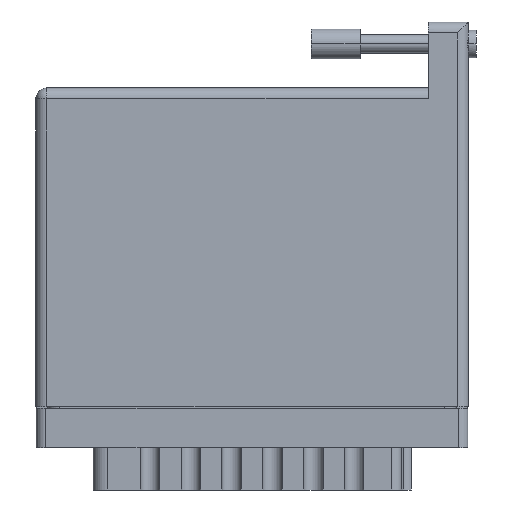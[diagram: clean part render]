
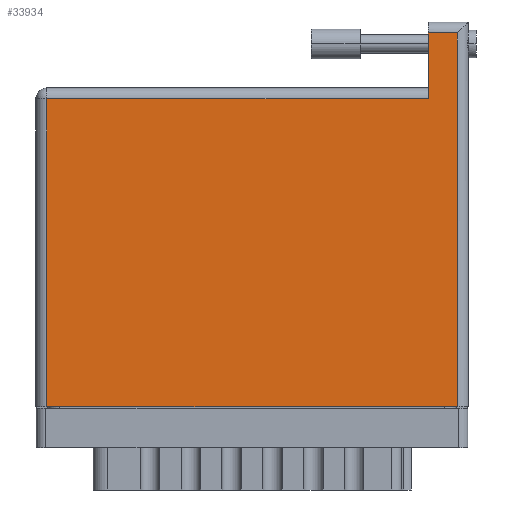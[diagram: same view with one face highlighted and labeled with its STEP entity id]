
A CAD part, front view. The second image highlights one B-rep face of the part: STEP entity #33934.
In plain terms, the highlighted face is planar.
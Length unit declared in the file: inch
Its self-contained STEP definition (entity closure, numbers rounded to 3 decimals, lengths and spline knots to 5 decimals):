
#3398 = CARTESIAN_POINT ( 'NONE',  ( 0., 2.38, 0. ) ) ;
#4438 = ORIENTED_EDGE ( 'NONE', *, *, #32680, .T. ) ;
#5184 = AXIS2_PLACEMENT_3D ( 'NONE', #55172, #81956, #68288 ) ;
#7127 = EDGE_CURVE ( 'NONE', #17863, #19327, #41618, .T. ) ;
#8335 = PLANE ( 'NONE',  #5184 ) ;
#9210 = VERTEX_POINT ( 'NONE', #64380 ) ;
#9655 = ORIENTED_EDGE ( 'NONE', *, *, #7127, .T. ) ;
#12893 = DIRECTION ( 'NONE',  ( 0., -1., 0. ) ) ;
#14380 = ORIENTED_EDGE ( 'NONE', *, *, #60143, .T. ) ;
#15387 = EDGE_LOOP ( 'NONE', ( #14380, #84192, #4438, #9655, #59409, #62923 ) ) ;
#15665 = CARTESIAN_POINT ( 'NONE',  ( 2.685, 0., 0. ) ) ;
#17863 = VERTEX_POINT ( 'NONE', #59185 ) ;
#19327 = VERTEX_POINT ( 'NONE', #15665 ) ;
#20785 = VECTOR ( 'NONE', #63947, 39.37008 ) ;
#22750 = CARTESIAN_POINT ( 'NONE',  ( 2.685, 2.38, 0. ) ) ;
#22816 = VECTOR ( 'NONE', #77597, 39.37008 ) ;
#23633 = CARTESIAN_POINT ( 'NONE',  ( 2.499, 1.96, 0. ) ) ;
#29413 = LINE ( 'NONE', #57463, #50228 ) ;
#31864 = CARTESIAN_POINT ( 'NONE',  ( 0., 0., 0. ) ) ;
#32680 = EDGE_CURVE ( 'NONE', #81911, #17863, #42531, .T. ) ;
#33247 = EDGE_CURVE ( 'NONE', #19327, #50905, #82071, .T. ) ;
#33934 = ADVANCED_FACE ( 'NONE', ( #63229 ), #8335, .F. ) ;
#36500 = DIRECTION ( 'NONE',  ( 0., -1., 0. ) ) ;
#39811 = DIRECTION ( 'NONE',  ( 0., 1., 0. ) ) ;
#41059 = VERTEX_POINT ( 'NONE', #23633 ) ;
#41294 = LINE ( 'NONE', #53736, #79901 ) ;
#41618 = LINE ( 'NONE', #31864, #22816 ) ;
#42531 = LINE ( 'NONE', #79247, #77936 ) ;
#46862 = LINE ( 'NONE', #3398, #20785 ) ;
#50228 = VECTOR ( 'NONE', #36500, 39.37008 ) ;
#50905 = VERTEX_POINT ( 'NONE', #22750 ) ;
#53736 = CARTESIAN_POINT ( 'NONE',  ( 0., 1.96, 0. ) ) ;
#54991 = EDGE_CURVE ( 'NONE', #50905, #9210, #46862, .T. ) ;
#55172 = CARTESIAN_POINT ( 'NONE',  ( 0., 2.03, 0. ) ) ;
#57463 = CARTESIAN_POINT ( 'NONE',  ( 2.499, 2.45, 0. ) ) ;
#59185 = CARTESIAN_POINT ( 'NONE',  ( 0.07, 0., 0. ) ) ;
#59409 = ORIENTED_EDGE ( 'NONE', *, *, #33247, .T. ) ;
#60143 = EDGE_CURVE ( 'NONE', #9210, #41059, #29413, .T. ) ;
#62923 = ORIENTED_EDGE ( 'NONE', *, *, #54991, .T. ) ;
#63229 = FACE_OUTER_BOUND ( 'NONE', #15387, .T. ) ;
#63947 = DIRECTION ( 'NONE',  ( -1., 0., 0. ) ) ;
#64141 = EDGE_CURVE ( 'NONE', #41059, #81911, #41294, .T. ) ;
#64380 = CARTESIAN_POINT ( 'NONE',  ( 2.499, 2.38, 0. ) ) ;
#64382 = VECTOR ( 'NONE', #39811, 39.37008 ) ;
#68288 = DIRECTION ( 'NONE',  ( -1., 0., 0. ) ) ;
#73569 = CARTESIAN_POINT ( 'NONE',  ( 2.685, 2.45, 0. ) ) ;
#76457 = CARTESIAN_POINT ( 'NONE',  ( 0.07, 1.96, 0. ) ) ;
#77597 = DIRECTION ( 'NONE',  ( 1., 0., 0. ) ) ;
#77936 = VECTOR ( 'NONE', #12893, 39.37008 ) ;
#79247 = CARTESIAN_POINT ( 'NONE',  ( 0.07, 0., 0. ) ) ;
#79901 = VECTOR ( 'NONE', #80518, 39.37008 ) ;
#80518 = DIRECTION ( 'NONE',  ( -1., 0., 0. ) ) ;
#81911 = VERTEX_POINT ( 'NONE', #76457 ) ;
#81956 = DIRECTION ( 'NONE',  ( 0., 0., -1. ) ) ;
#82071 = LINE ( 'NONE', #73569, #64382 ) ;
#84192 = ORIENTED_EDGE ( 'NONE', *, *, #64141, .T. ) ;
